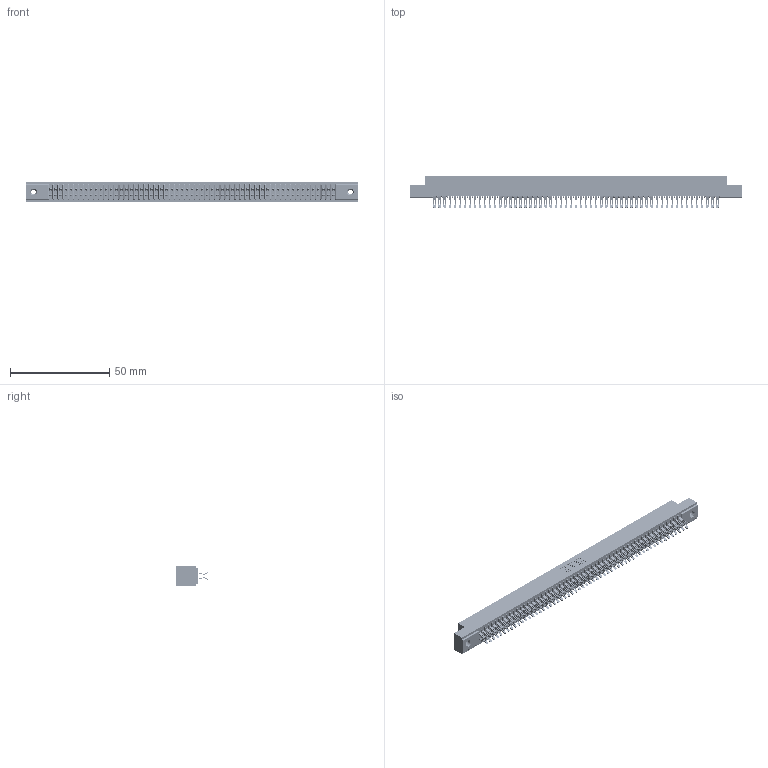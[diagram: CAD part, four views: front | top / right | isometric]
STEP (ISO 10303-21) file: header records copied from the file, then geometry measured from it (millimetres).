
FILE_DESCRIPTION (( 'STEP AP203' ), '1' );
FILE_NAME ('341-114-555-208.STEP', '2018-08-08T13:40:10', ( '' ), ( '' ), 'SwSTEP 2.0', 'SolidWorks 2016', '' );
FILE_SCHEMA (( 'CONFIG_CONTROL_DESIGN' ));
Length unit declared in the file: inch
Products named in the file (4): 341 Part_.156 (3.96) Dia Mounting Holes; 341-292-001_341-292-155; 345-250-001_345-250-003-102; 341-114-555-208
Assembly tree (117 placements, depth 2):
  341-114-555-208
    341 Part_.156 (3.96) Dia Mounting Holes
    341-292-001_341-292-155  x114
    345-250-001_345-250-003-102  x2
Bounding box: 167 x 16.31 x 10.16 mm (x, y, z)
Volume: 12484.1 mm3; surface area: 23583.5 mm2
Topology: 117 solids, 117 shells, 9068 faces, 27071 edges, 17618 vertices
Faces by surface type: plane 4888, cylinder 3936, sphere 116, torus 116, cone 12
Entity records: 68639 total; most frequent: CARTESIAN_POINT 11408, ORIENTED_EDGE 11322, DIRECTION 11061, EDGE_CURVE 5661, VECTOR 4571, LINE 4571, VERTEX_POINT 3576, AXIS2_PLACEMENT_3D 3245
